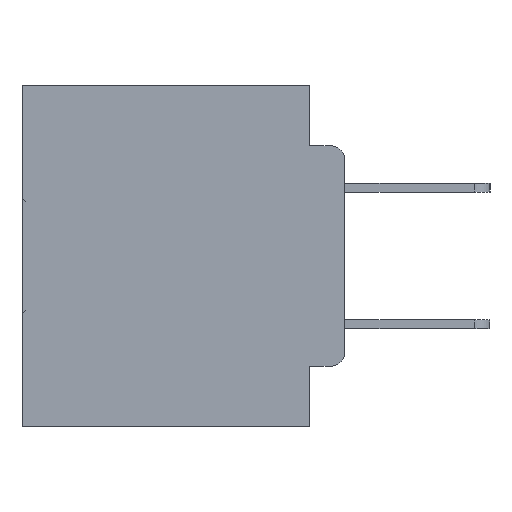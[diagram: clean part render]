
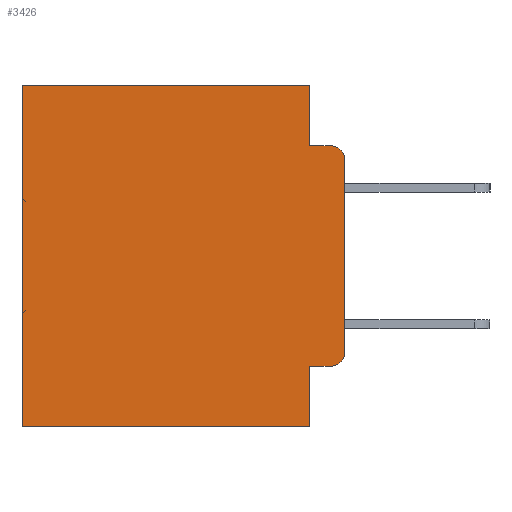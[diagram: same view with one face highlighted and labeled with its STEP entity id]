
A CAD part, left-side view. The second image highlights one B-rep face of the part: STEP entity #3426.
In plain terms, the highlighted planar face has unit normal (-1, 0, 0).
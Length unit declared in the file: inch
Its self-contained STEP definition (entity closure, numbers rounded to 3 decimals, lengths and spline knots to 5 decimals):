
#2241 = ORIENTED_EDGE ( 'NONE', *, *, #30769, .T. ) ;
#2365 = CARTESIAN_POINT ( 'NONE',  ( 0.298, 0., -0.5 ) ) ;
#2655 = VERTEX_POINT ( 'NONE', #12701 ) ;
#3426 = ADVANCED_FACE ( 'NONE', ( #11230 ), #10963, .F. ) ;
#3786 = CARTESIAN_POINT ( 'NONE',  ( 0.298, 0., 0. ) ) ;
#3992 = EDGE_CURVE ( 'NONE', #16529, #19388, #10355, .T. ) ;
#4008 = AXIS2_PLACEMENT_3D ( 'NONE', #15076, #33451, #17748 ) ;
#4668 = CARTESIAN_POINT ( 'NONE',  ( 0.298, 0.02, -0.4115 ) ) ;
#4743 = VECTOR ( 'NONE', #22602, 39.37008 ) ;
#4943 = DIRECTION ( 'NONE',  ( 0., 1., 0. ) ) ;
#5463 = CARTESIAN_POINT ( 'NONE',  ( 0.298, 0.051, -0.0885 ) ) ;
#5727 = CARTESIAN_POINT ( 'NONE',  ( 0.298, 0.473, -0.5 ) ) ;
#6022 = ORIENTED_EDGE ( 'NONE', *, *, #26506, .F. ) ;
#7259 = CARTESIAN_POINT ( 'NONE',  ( 0.298, 0.02, -0.1085 ) ) ;
#7348 = ORIENTED_EDGE ( 'NONE', *, *, #17111, .F. ) ;
#7736 = ORIENTED_EDGE ( 'NONE', *, *, #32047, .F. ) ;
#8005 = DIRECTION ( 'NONE',  ( 0., 0., -1. ) ) ;
#8061 = CARTESIAN_POINT ( 'NONE',  ( 0.298, 0.051, 0. ) ) ;
#9464 = EDGE_CURVE ( 'NONE', #34208, #26845, #11897, .T. ) ;
#9638 = EDGE_LOOP ( 'NONE', ( #25667, #14417, #26866, #7348, #2241, #11085, #6022, #7736, #14087, #11183 ) ) ;
#9939 = DIRECTION ( 'NONE',  ( 0., 0., -1. ) ) ;
#10350 = CARTESIAN_POINT ( 'NONE',  ( 0.298, 0., 0. ) ) ;
#10352 = LINE ( 'NONE', #10350, #28975 ) ;
#10355 = LINE ( 'NONE', #19641, #15758 ) ;
#10470 = DIRECTION ( 'NONE',  ( 0., 1., 0. ) ) ;
#10729 = DIRECTION ( 'NONE',  ( 0., 0., -1. ) ) ;
#10791 = EDGE_CURVE ( 'NONE', #34208, #27176, #31204, .T. ) ;
#10848 = DIRECTION ( 'NONE',  ( 1., 0., 0. ) ) ;
#10963 = PLANE ( 'NONE',  #13518 ) ;
#11085 = ORIENTED_EDGE ( 'NONE', *, *, #3992, .T. ) ;
#11183 = ORIENTED_EDGE ( 'NONE', *, *, #14717, .T. ) ;
#11230 = FACE_OUTER_BOUND ( 'NONE', #9638, .T. ) ;
#11897 = LINE ( 'NONE', #3786, #4743 ) ;
#12701 = CARTESIAN_POINT ( 'NONE',  ( 0.298, 0.051, -0.5 ) ) ;
#13006 = VECTOR ( 'NONE', #25941, 39.37008 ) ;
#13518 = AXIS2_PLACEMENT_3D ( 'NONE', #21912, #10848, #10729 ) ;
#14003 = LINE ( 'NONE', #31981, #21935 ) ;
#14087 = ORIENTED_EDGE ( 'NONE', *, *, #28875, .T. ) ;
#14417 = ORIENTED_EDGE ( 'NONE', *, *, #10791, .T. ) ;
#14717 = EDGE_CURVE ( 'NONE', #31881, #26845, #31991, .T. ) ;
#15009 = LINE ( 'NONE', #27955, #22096 ) ;
#15076 = CARTESIAN_POINT ( 'NONE',  ( 0.298, 0.02, -0.3915 ) ) ;
#15362 = DIRECTION ( 'NONE',  ( 0., -1., 0. ) ) ;
#15758 = VECTOR ( 'NONE', #8005, 39.37008 ) ;
#16020 = CARTESIAN_POINT ( 'NONE',  ( 0.298, 0.02, -0.0885 ) ) ;
#16250 = AXIS2_PLACEMENT_3D ( 'NONE', #7259, #25867, #9939 ) ;
#16529 = VERTEX_POINT ( 'NONE', #22546 ) ;
#17111 = EDGE_CURVE ( 'NONE', #30196, #21055, #15009, .T. ) ;
#17315 = CARTESIAN_POINT ( 'NONE',  ( 0.298, 0., -0.3915 ) ) ;
#17429 = LINE ( 'NONE', #2365, #23675 ) ;
#17748 = DIRECTION ( 'NONE',  ( 0., 0., -1. ) ) ;
#18584 = EDGE_CURVE ( 'NONE', #21055, #27176, #25730, .T. ) ;
#19239 = LINE ( 'NONE', #23287, #13006 ) ;
#19388 = VERTEX_POINT ( 'NONE', #5727 ) ;
#19641 = CARTESIAN_POINT ( 'NONE',  ( 0.298, 0.473, 0. ) ) ;
#21055 = VERTEX_POINT ( 'NONE', #5463 ) ;
#21347 = VERTEX_POINT ( 'NONE', #22743 ) ;
#21502 = DIRECTION ( 'NONE',  ( 0., 0., -1. ) ) ;
#21912 = CARTESIAN_POINT ( 'NONE',  ( 0.298, 0., 0. ) ) ;
#21935 = VECTOR ( 'NONE', #21502, 39.37008 ) ;
#22096 = VECTOR ( 'NONE', #33038, 39.37008 ) ;
#22546 = CARTESIAN_POINT ( 'NONE',  ( 0.298, 0.473, 0. ) ) ;
#22602 = DIRECTION ( 'NONE',  ( 0., 0., -1. ) ) ;
#22743 = CARTESIAN_POINT ( 'NONE',  ( 0.298, 0.051, -0.4115 ) ) ;
#23002 = CARTESIAN_POINT ( 'NONE',  ( 0.298, 0., -0.1085 ) ) ;
#23287 = CARTESIAN_POINT ( 'NONE',  ( 0.298, 0.051, -0.4115 ) ) ;
#23675 = VECTOR ( 'NONE', #10470, 39.37008 ) ;
#25667 = ORIENTED_EDGE ( 'NONE', *, *, #9464, .F. ) ;
#25730 = LINE ( 'NONE', #33739, #31786 ) ;
#25867 = DIRECTION ( 'NONE',  ( -1., 0., 0. ) ) ;
#25941 = DIRECTION ( 'NONE',  ( 0., -1., 0. ) ) ;
#26506 = EDGE_CURVE ( 'NONE', #2655, #19388, #17429, .T. ) ;
#26845 = VERTEX_POINT ( 'NONE', #17315 ) ;
#26866 = ORIENTED_EDGE ( 'NONE', *, *, #18584, .F. ) ;
#27176 = VERTEX_POINT ( 'NONE', #16020 ) ;
#27955 = CARTESIAN_POINT ( 'NONE',  ( 0.298, 0.051, 0. ) ) ;
#28875 = EDGE_CURVE ( 'NONE', #21347, #31881, #19239, .T. ) ;
#28975 = VECTOR ( 'NONE', #4943, 39.37008 ) ;
#30196 = VERTEX_POINT ( 'NONE', #8061 ) ;
#30769 = EDGE_CURVE ( 'NONE', #30196, #16529, #10352, .T. ) ;
#31204 = CIRCLE ( 'NONE', #16250, 0.02 ) ;
#31786 = VECTOR ( 'NONE', #15362, 39.37008 ) ;
#31881 = VERTEX_POINT ( 'NONE', #4668 ) ;
#31981 = CARTESIAN_POINT ( 'NONE',  ( 0.298, 0.051, 0. ) ) ;
#31991 = CIRCLE ( 'NONE', #4008, 0.02 ) ;
#32047 = EDGE_CURVE ( 'NONE', #21347, #2655, #14003, .T. ) ;
#33038 = DIRECTION ( 'NONE',  ( 0., 0., -1. ) ) ;
#33451 = DIRECTION ( 'NONE',  ( -1., 0., 0. ) ) ;
#33739 = CARTESIAN_POINT ( 'NONE',  ( 0.298, 0.051, -0.0885 ) ) ;
#34208 = VERTEX_POINT ( 'NONE', #23002 ) ;
